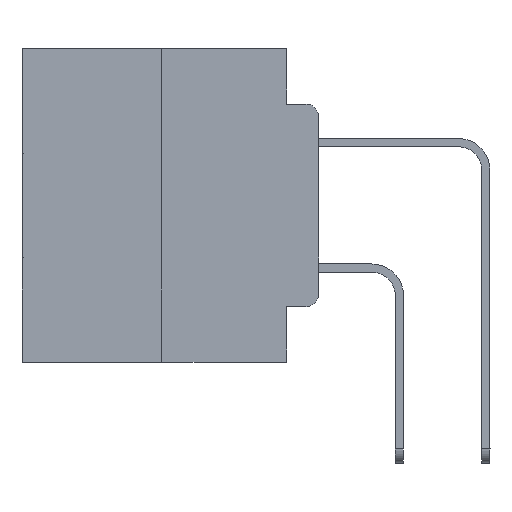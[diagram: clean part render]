
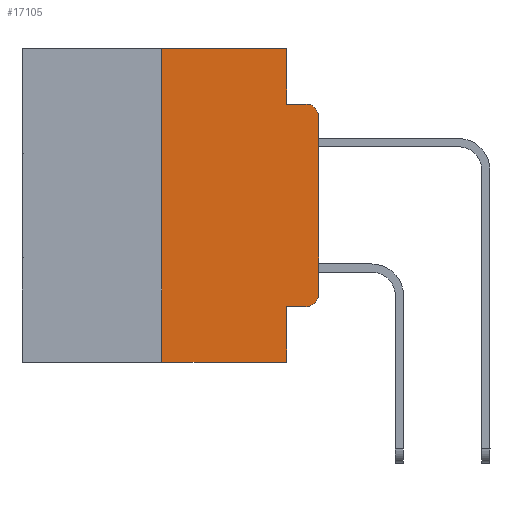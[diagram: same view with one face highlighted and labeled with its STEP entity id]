
A CAD part, left-side view. The second image highlights one B-rep face of the part: STEP entity #17105.
In plain terms, the highlighted planar face has unit normal (-1, 0, 0).
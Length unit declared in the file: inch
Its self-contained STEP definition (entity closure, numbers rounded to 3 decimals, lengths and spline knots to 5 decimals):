
#44 = EDGE_CURVE ( 'NONE', #20854, #11858, #21310, .T. ) ;
#144 = VECTOR ( 'NONE', #10083, 39.37008 ) ;
#174 = CARTESIAN_POINT ( 'NONE',  ( 0., 0.051, 0. ) ) ;
#382 = CARTESIAN_POINT ( 'NONE',  ( 0., 0.051, -0.4115 ) ) ;
#496 = CARTESIAN_POINT ( 'NONE',  ( 0., 0.473, 0. ) ) ;
#562 = LINE ( 'NONE', #28962, #144 ) ;
#590 = DIRECTION ( 'NONE',  ( -1., 0., 0. ) ) ;
#987 = LINE ( 'NONE', #8158, #3382 ) ;
#2090 = DIRECTION ( 'NONE',  ( 0., 0., -1. ) ) ;
#2632 = CARTESIAN_POINT ( 'NONE',  ( 0., 0.02, -0.3915 ) ) ;
#3178 = EDGE_CURVE ( 'NONE', #20242, #15946, #6135, .T. ) ;
#3382 = VECTOR ( 'NONE', #29852, 39.37008 ) ;
#3600 = ORIENTED_EDGE ( 'NONE', *, *, #5563, .T. ) ;
#4024 = ORIENTED_EDGE ( 'NONE', *, *, #7269, .F. ) ;
#4648 = EDGE_CURVE ( 'NONE', #14344, #15946, #19067, .T. ) ;
#4866 = PLANE ( 'NONE',  #9921 ) ;
#4972 = DIRECTION ( 'NONE',  ( -1., 0., 0. ) ) ;
#5563 = EDGE_CURVE ( 'NONE', #14344, #10243, #14593, .T. ) ;
#6135 = LINE ( 'NONE', #22954, #28365 ) ;
#6170 = CARTESIAN_POINT ( 'NONE',  ( 0., 0.051, -0.4115 ) ) ;
#6182 = EDGE_CURVE ( 'NONE', #11858, #12705, #15618, .T. ) ;
#6190 = VECTOR ( 'NONE', #30586, 39.37008 ) ;
#6347 = CARTESIAN_POINT ( 'NONE',  ( 0., 0.051, -0.0885 ) ) ;
#6875 = AXIS2_PLACEMENT_3D ( 'NONE', #2632, #4972, #14655 ) ;
#7269 = EDGE_CURVE ( 'NONE', #20242, #20854, #28633, .T. ) ;
#7667 = CARTESIAN_POINT ( 'NONE',  ( 0., 0.02, -0.0885 ) ) ;
#7748 = CARTESIAN_POINT ( 'NONE',  ( 0., 0.25, -0.5 ) ) ;
#8158 = CARTESIAN_POINT ( 'NONE',  ( 0., 0., 0. ) ) ;
#8229 = EDGE_CURVE ( 'NONE', #16235, #17100, #13665, .T. ) ;
#9167 = VECTOR ( 'NONE', #9902, 39.37008 ) ;
#9475 = DIRECTION ( 'NONE',  ( 0., -1., 0. ) ) ;
#9902 = DIRECTION ( 'NONE',  ( 0., -1., 0. ) ) ;
#9921 = AXIS2_PLACEMENT_3D ( 'NONE', #496, #10018, #24338 ) ;
#10018 = DIRECTION ( 'NONE',  ( 1., 0., 0. ) ) ;
#10029 = VECTOR ( 'NONE', #25968, 39.37008 ) ;
#10083 = DIRECTION ( 'NONE',  ( 0., -1., 0. ) ) ;
#10243 = VERTEX_POINT ( 'NONE', #14857 ) ;
#10406 = VECTOR ( 'NONE', #2090, 39.37008 ) ;
#11106 = CARTESIAN_POINT ( 'NONE',  ( 0., 0.051, 0. ) ) ;
#11858 = VERTEX_POINT ( 'NONE', #174 ) ;
#12570 = CARTESIAN_POINT ( 'NONE',  ( 0., 0.25, 0. ) ) ;
#12705 = VERTEX_POINT ( 'NONE', #6347 ) ;
#13103 = ORIENTED_EDGE ( 'NONE', *, *, #6182, .F. ) ;
#13613 = ORIENTED_EDGE ( 'NONE', *, *, #22781, .F. ) ;
#13665 = CIRCLE ( 'NONE', #21589, 0.02 ) ;
#14200 = ORIENTED_EDGE ( 'NONE', *, *, #4648, .F. ) ;
#14344 = VERTEX_POINT ( 'NONE', #6170 ) ;
#14370 = EDGE_CURVE ( 'NONE', #10243, #20502, #17824, .T. ) ;
#14593 = LINE ( 'NONE', #382, #9167 ) ;
#14655 = DIRECTION ( 'NONE',  ( 0., 0., -1. ) ) ;
#14857 = CARTESIAN_POINT ( 'NONE',  ( 0., 0.02, -0.4115 ) ) ;
#14939 = CARTESIAN_POINT ( 'NONE',  ( 0., 0.02, -0.1085 ) ) ;
#15497 = EDGE_CURVE ( 'NONE', #20502, #16235, #987, .T. ) ;
#15618 = LINE ( 'NONE', #11106, #6190 ) ;
#15648 = DIRECTION ( 'NONE',  ( 0., -1., 0. ) ) ;
#15946 = VERTEX_POINT ( 'NONE', #27421 ) ;
#16235 = VERTEX_POINT ( 'NONE', #16954 ) ;
#16470 = CARTESIAN_POINT ( 'NONE',  ( 0., 0.25, 0. ) ) ;
#16954 = CARTESIAN_POINT ( 'NONE',  ( 0., 0., -0.1085 ) ) ;
#17100 = VERTEX_POINT ( 'NONE', #7667 ) ;
#17105 = ADVANCED_FACE ( 'NONE', ( #21839 ), #4866, .F. ) ;
#17824 = CIRCLE ( 'NONE', #6875, 0.02 ) ;
#19067 = LINE ( 'NONE', #28739, #10406 ) ;
#19134 = CARTESIAN_POINT ( 'NONE',  ( 0., 0.473, 0. ) ) ;
#19513 = ORIENTED_EDGE ( 'NONE', *, *, #14370, .T. ) ;
#20242 = VERTEX_POINT ( 'NONE', #7748 ) ;
#20502 = VERTEX_POINT ( 'NONE', #28019 ) ;
#20854 = VERTEX_POINT ( 'NONE', #12570 ) ;
#21310 = LINE ( 'NONE', #19134, #22640 ) ;
#21589 = AXIS2_PLACEMENT_3D ( 'NONE', #14939, #590, #21928 ) ;
#21839 = FACE_OUTER_BOUND ( 'NONE', #25124, .T. ) ;
#21928 = DIRECTION ( 'NONE',  ( 0., 0., -1. ) ) ;
#22640 = VECTOR ( 'NONE', #9475, 39.37008 ) ;
#22781 = EDGE_CURVE ( 'NONE', #12705, #17100, #562, .T. ) ;
#22954 = CARTESIAN_POINT ( 'NONE',  ( 0., 0.473, -0.5 ) ) ;
#24090 = ORIENTED_EDGE ( 'NONE', *, *, #8229, .T. ) ;
#24338 = DIRECTION ( 'NONE',  ( 0., 0., -1. ) ) ;
#25124 = EDGE_LOOP ( 'NONE', ( #30389, #24090, #13613, #13103, #27853, #4024, #27653, #14200, #3600, #19513 ) ) ;
#25968 = DIRECTION ( 'NONE',  ( 0., 0., 1. ) ) ;
#27421 = CARTESIAN_POINT ( 'NONE',  ( 0., 0.051, -0.5 ) ) ;
#27653 = ORIENTED_EDGE ( 'NONE', *, *, #3178, .T. ) ;
#27853 = ORIENTED_EDGE ( 'NONE', *, *, #44, .F. ) ;
#28019 = CARTESIAN_POINT ( 'NONE',  ( 0., 0., -0.3915 ) ) ;
#28365 = VECTOR ( 'NONE', #15648, 39.37008 ) ;
#28633 = LINE ( 'NONE', #16470, #10029 ) ;
#28739 = CARTESIAN_POINT ( 'NONE',  ( 0., 0.051, 0. ) ) ;
#28962 = CARTESIAN_POINT ( 'NONE',  ( 0., 0.051, -0.0885 ) ) ;
#29852 = DIRECTION ( 'NONE',  ( 0., 0., 1. ) ) ;
#30389 = ORIENTED_EDGE ( 'NONE', *, *, #15497, .T. ) ;
#30586 = DIRECTION ( 'NONE',  ( 0., 0., -1. ) ) ;
